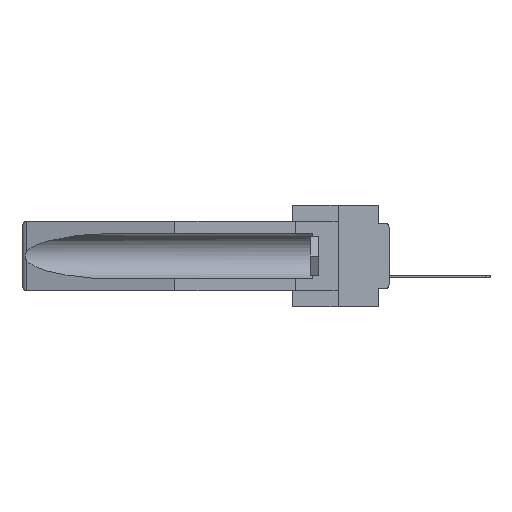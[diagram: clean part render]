
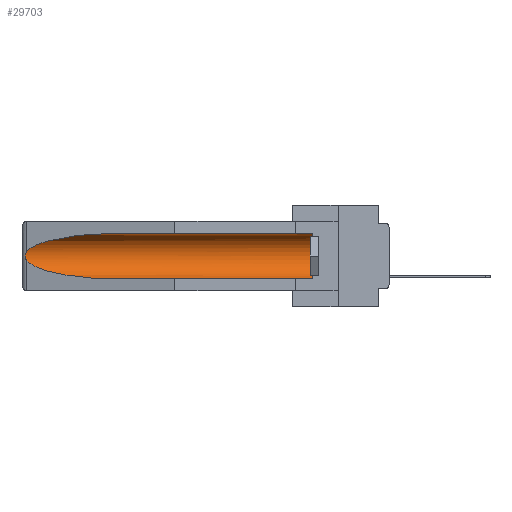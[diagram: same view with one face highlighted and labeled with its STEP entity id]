
A CAD part, left-side view. The second image highlights one B-rep face of the part: STEP entity #29703.
In plain terms, the highlighted cylindrical face has radius 2.857 mm (diameter 5.715 mm), a partial arc.
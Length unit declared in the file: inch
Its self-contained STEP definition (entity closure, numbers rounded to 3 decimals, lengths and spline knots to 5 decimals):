
#862 = CARTESIAN_POINT ( 'NONE',  ( 0.155, -0.30754, -0.284 ) ) ;
#899 = CARTESIAN_POINT ( 'NONE',  ( 0.25451, 1.48313, -0.24835 ) ) ;
#1166 = DIRECTION ( 'NONE',  ( 0., -1., 0. ) ) ;
#1707 = CARTESIAN_POINT ( 'NONE',  ( 0.155, -0.30754, -0.1715 ) ) ;
#2690 = CARTESIAN_POINT ( 'NONE',  ( 0.26537, 1.52718, -0.19328 ) ) ;
#3010 = CARTESIAN_POINT ( 'NONE',  ( 0.155, 1.07973, -0.059 ) ) ;
#3146 = ORIENTED_EDGE ( 'NONE', *, *, #15171, .T. ) ;
#4693 = FACE_OUTER_BOUND ( 'NONE', #18399, .T. ) ;
#4832 = CARTESIAN_POINT ( 'NONE',  ( 0.26537, 1.52718, -0.19328 ) ) ;
#5933 = EDGE_CURVE ( 'NONE', #18027, #30729, #25547, .T. ) ;
#6909 = DIRECTION ( 'NONE',  ( 0., 1., 0. ) ) ;
#7320 = EDGE_CURVE ( 'NONE', #22601, #19083, #29718, .T. ) ;
#8431 = AXIS2_PLACEMENT_3D ( 'NONE', #1707, #15245, #9987 ) ;
#8598 = CARTESIAN_POINT ( 'NONE',  ( 0.155, 0.126, -0.1715 ) ) ;
#9697 = CARTESIAN_POINT ( 'NONE',  ( 0.21114, 1.30732, -0.059 ) ) ;
#9955 =( BOUNDED_CURVE ( )  B_SPLINE_CURVE ( 3, ( #17625, #9697, #22563, #27997 ),
 .UNSPECIFIED., .F., .T. ) 
 B_SPLINE_CURVE_WITH_KNOTS ( ( 4, 4 ),
 ( 4.71239, 6.08839 ),
 .UNSPECIFIED. ) 
 CURVE ( )  GEOMETRIC_REPRESENTATION_ITEM ( )  RATIONAL_B_SPLINE_CURVE ( ( 1., 0.848, 0.848, 1. ) ) 
 REPRESENTATION_ITEM ( '' )  );
#9987 = DIRECTION ( 'NONE',  ( 0., 0., 1. ) ) ;
#10472 = CARTESIAN_POINT ( 'NONE',  ( 0.2675, 1.53308, -0.16763 ) ) ;
#11305 = CARTESIAN_POINT ( 'NONE',  ( 0.155, 1.07973, -0.284 ) ) ;
#11524 = ORIENTED_EDGE ( 'NONE', *, *, #17112, .T. ) ;
#12178 = ORIENTED_EDGE ( 'NONE', *, *, #20528, .T. ) ;
#14202 = CARTESIAN_POINT ( 'NONE',  ( 0.155, 0.126, -0.059 ) ) ;
#15171 = EDGE_CURVE ( 'NONE', #22601, #18027, #17701, .T. ) ;
#15245 = DIRECTION ( 'NONE',  ( 0., 1., 0. ) ) ;
#15516 = CARTESIAN_POINT ( 'NONE',  ( 0.155, 1.07973, -0.284 ) ) ;
#15727 = CARTESIAN_POINT ( 'NONE',  ( 0.26597, 1.5296, -0.19026 ) ) ;
#17112 = EDGE_CURVE ( 'NONE', #20926, #33167, #18963, .T. ) ;
#17625 = CARTESIAN_POINT ( 'NONE',  ( 0.155, 1.07973, -0.059 ) ) ;
#17701 = CIRCLE ( 'NONE', #32264, 0.1125 ) ;
#18027 = VERTEX_POINT ( 'NONE', #14202 ) ;
#18399 = EDGE_LOOP ( 'NONE', ( #34496, #11524, #12178, #33471, #3146, #29609 ) ) ;
#18963 = B_SPLINE_CURVE_WITH_KNOTS ( 'NONE', 3,
 ( #21372, #28924, #29615, #31903, #10472, #23663, #32243, #29267, #15727, #4832 ),
 .UNSPECIFIED., .F., .F.,
 ( 4, 2, 2, 2, 4 ),
 ( 0., 0.00029, 0.00058, 0.00087, 0.00117 ),
 .UNSPECIFIED. ) ;
#19016 = DIRECTION ( 'NONE',  ( 0., 1., 0. ) ) ;
#19083 = VERTEX_POINT ( 'NONE', #15516 ) ;
#20528 = EDGE_CURVE ( 'NONE', #33167, #19083, #29258, .T. ) ;
#20926 = VERTEX_POINT ( 'NONE', #21297 ) ;
#21136 = VECTOR ( 'NONE', #6909, 39.37008 ) ;
#21297 = CARTESIAN_POINT ( 'NONE',  ( 0.26537, 1.52718, -0.14972 ) ) ;
#21372 = CARTESIAN_POINT ( 'NONE',  ( 0.26537, 1.52718, -0.14972 ) ) ;
#22138 = DIRECTION ( 'NONE',  ( 0., 0., 1. ) ) ;
#22563 = CARTESIAN_POINT ( 'NONE',  ( 0.25451, 1.48313, -0.09465 ) ) ;
#22601 = VERTEX_POINT ( 'NONE', #31535 ) ;
#22809 = EDGE_CURVE ( 'NONE', #30729, #20926, #9955, .T. ) ;
#23663 = CARTESIAN_POINT ( 'NONE',  ( 0.2675, 1.53308, -0.17534 ) ) ;
#25547 = LINE ( 'NONE', #30981, #21136 ) ;
#25820 = CYLINDRICAL_SURFACE ( 'NONE', #8431, 0.1125 ) ;
#27997 = CARTESIAN_POINT ( 'NONE',  ( 0.26537, 1.52718, -0.14972 ) ) ;
#28924 = CARTESIAN_POINT ( 'NONE',  ( 0.26597, 1.52961, -0.15275 ) ) ;
#29258 =( BOUNDED_CURVE ( )  B_SPLINE_CURVE ( 3, ( #33253, #899, #30106, #11305 ),
 .UNSPECIFIED., .F., .T. ) 
 B_SPLINE_CURVE_WITH_KNOTS ( ( 4, 4 ),
 ( 0.1948, 1.5708 ),
 .UNSPECIFIED. ) 
 CURVE ( )  GEOMETRIC_REPRESENTATION_ITEM ( )  RATIONAL_B_SPLINE_CURVE ( ( 1., 0.848, 0.848, 1. ) ) 
 REPRESENTATION_ITEM ( '' )  );
#29267 = CARTESIAN_POINT ( 'NONE',  ( 0.26655, 1.53094, -0.18657 ) ) ;
#29609 = ORIENTED_EDGE ( 'NONE', *, *, #5933, .T. ) ;
#29615 = CARTESIAN_POINT ( 'NONE',  ( 0.26654, 1.53092, -0.15636 ) ) ;
#29703 = ADVANCED_FACE ( 'NONE', ( #4693 ), #25820, .F. ) ;
#29718 = LINE ( 'NONE', #862, #34288 ) ;
#30106 = CARTESIAN_POINT ( 'NONE',  ( 0.21114, 1.30732, -0.284 ) ) ;
#30729 = VERTEX_POINT ( 'NONE', #3010 ) ;
#30981 = CARTESIAN_POINT ( 'NONE',  ( 0.155, -0.30754, -0.059 ) ) ;
#31535 = CARTESIAN_POINT ( 'NONE',  ( 0.155, 0.126, -0.284 ) ) ;
#31903 = CARTESIAN_POINT ( 'NONE',  ( 0.2673, 1.5327, -0.16383 ) ) ;
#32243 = CARTESIAN_POINT ( 'NONE',  ( 0.2673, 1.53269, -0.17917 ) ) ;
#32264 = AXIS2_PLACEMENT_3D ( 'NONE', #8598, #1166, #22138 ) ;
#33167 = VERTEX_POINT ( 'NONE', #2690 ) ;
#33253 = CARTESIAN_POINT ( 'NONE',  ( 0.26537, 1.52718, -0.19328 ) ) ;
#33471 = ORIENTED_EDGE ( 'NONE', *, *, #7320, .F. ) ;
#34288 = VECTOR ( 'NONE', #19016, 39.37008 ) ;
#34496 = ORIENTED_EDGE ( 'NONE', *, *, #22809, .T. ) ;
